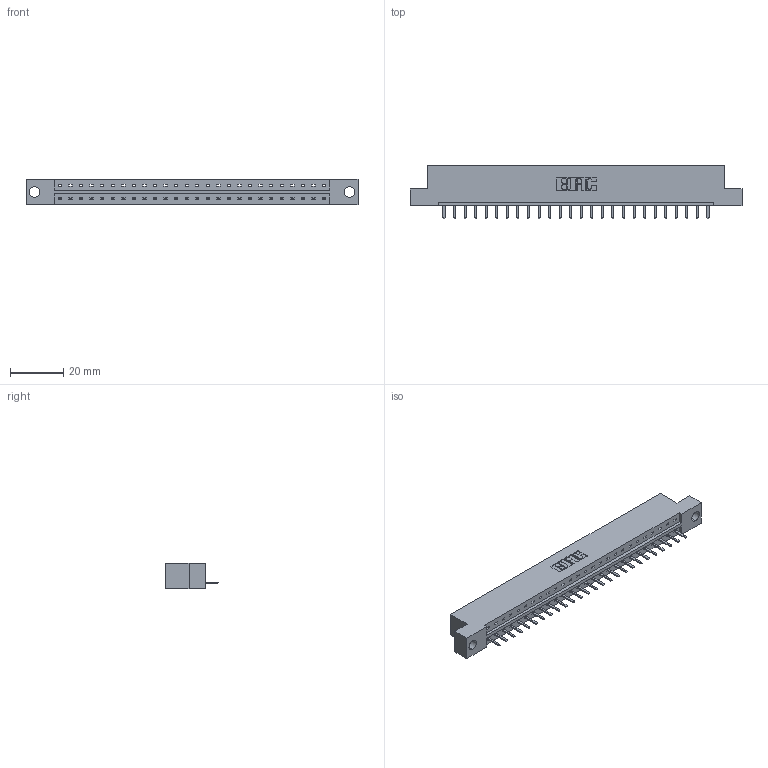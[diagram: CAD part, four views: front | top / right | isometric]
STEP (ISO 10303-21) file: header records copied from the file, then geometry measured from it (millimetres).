
FILE_DESCRIPTION (( 'STEP AP203' ), '1' );
FILE_NAME ('333-026-520-104.STEP', '2018-08-02T12:28:52', ( '' ), ( '' ), 'SwSTEP 2.0', 'SolidWorks 2016', '' );
FILE_SCHEMA (( 'CONFIG_CONTROL_DESIGN' ));
Length unit declared in the file: inch
Products named in the file (3): 333 Part_Flush - .156 Dia - TH; 345-292-001_345-293-120; 333-026-520-104
Assembly tree (27 placements, depth 2):
  333-026-520-104
    333 Part_Flush - .156 Dia - TH
    345-292-001_345-293-120  x26
Bounding box: 124.56 x 20.02 x 9.4 mm (x, y, z)
Volume: 12234.2 mm3; surface area: 12665.5 mm2
Topology: 27 solids, 27 shells, 1726 faces, 5095 edges, 3326 vertices
Faces by surface type: plane 1214, cylinder 512
Entity records: 18081 total; most frequent: CARTESIAN_POINT 3140, ORIENTED_EDGE 3090, DIRECTION 2669, EDGE_CURVE 1545, VECTOR 1413, LINE 1413, VERTEX_POINT 1026, AXIS2_PLACEMENT_3D 628
